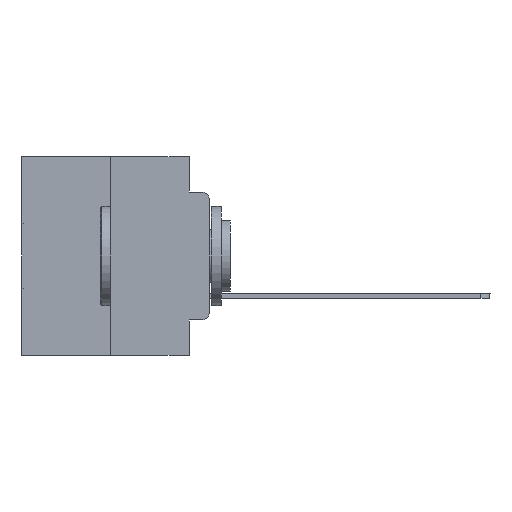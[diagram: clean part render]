
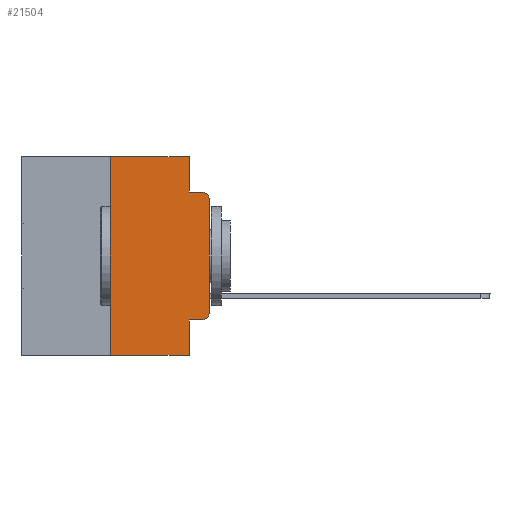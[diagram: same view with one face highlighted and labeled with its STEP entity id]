
A CAD part, left-side view. The second image highlights one B-rep face of the part: STEP entity #21504.
In plain terms, the highlighted planar face has unit normal (-1, 0, 0).
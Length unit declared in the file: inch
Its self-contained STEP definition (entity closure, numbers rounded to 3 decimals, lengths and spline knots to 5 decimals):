
#496 = VERTEX_POINT ( 'NONE', #14331 ) ;
#575 = EDGE_CURVE ( 'NONE', #27994, #496, #18154, .T. ) ;
#603 = ORIENTED_EDGE ( 'NONE', *, *, #17775, .T. ) ;
#1297 = CARTESIAN_POINT ( 'NONE',  ( 0., 0.473, 0. ) ) ;
#1309 = EDGE_CURVE ( 'NONE', #20811, #4275, #5692, .T. ) ;
#1399 = CARTESIAN_POINT ( 'NONE',  ( 0., 0.473, -0.5 ) ) ;
#2250 = EDGE_CURVE ( 'NONE', #29771, #3400, #20790, .T. ) ;
#2558 = CARTESIAN_POINT ( 'NONE',  ( 0., 0.02, -0.0885 ) ) ;
#2695 = VECTOR ( 'NONE', #11260, 39.37008 ) ;
#2806 = VECTOR ( 'NONE', #29273, 39.37008 ) ;
#2868 = ORIENTED_EDGE ( 'NONE', *, *, #575, .F. ) ;
#3094 = ORIENTED_EDGE ( 'NONE', *, *, #13580, .T. ) ;
#3380 = DIRECTION ( 'NONE',  ( 0., 0., -1. ) ) ;
#3400 = VERTEX_POINT ( 'NONE', #21935 ) ;
#3693 = DIRECTION ( 'NONE',  ( 0., -1., 0. ) ) ;
#4275 = VERTEX_POINT ( 'NONE', #17521 ) ;
#4934 = CARTESIAN_POINT ( 'NONE',  ( 0., 0.051, -0.0885 ) ) ;
#5692 = LINE ( 'NONE', #26639, #30234 ) ;
#5928 = DIRECTION ( 'NONE',  ( 0., 0., -1. ) ) ;
#6396 = VECTOR ( 'NONE', #3380, 39.37008 ) ;
#7435 = ORIENTED_EDGE ( 'NONE', *, *, #1309, .F. ) ;
#7499 = ORIENTED_EDGE ( 'NONE', *, *, #9379, .F. ) ;
#7923 = VERTEX_POINT ( 'NONE', #25984 ) ;
#8230 = CARTESIAN_POINT ( 'NONE',  ( 0., 0.051, 0. ) ) ;
#8682 = VERTEX_POINT ( 'NONE', #19244 ) ;
#9379 = EDGE_CURVE ( 'NONE', #8682, #20811, #21922, .T. ) ;
#9762 = ORIENTED_EDGE ( 'NONE', *, *, #10358, .F. ) ;
#10358 = EDGE_CURVE ( 'NONE', #18002, #27640, #24179, .T. ) ;
#10491 = LINE ( 'NONE', #1399, #2806 ) ;
#10536 = FACE_OUTER_BOUND ( 'NONE', #30091, .T. ) ;
#10923 = LINE ( 'NONE', #24789, #18863 ) ;
#11260 = DIRECTION ( 'NONE',  ( 0., 0., 1. ) ) ;
#11523 = ORIENTED_EDGE ( 'NONE', *, *, #27956, .F. ) ;
#13169 = CARTESIAN_POINT ( 'NONE',  ( 0., 0.051, -0.4115 ) ) ;
#13470 = DIRECTION ( 'NONE',  ( 0., 0., -1. ) ) ;
#13580 = EDGE_CURVE ( 'NONE', #27994, #7923, #10923, .T. ) ;
#14300 = VECTOR ( 'NONE', #17099, 39.37008 ) ;
#14331 = CARTESIAN_POINT ( 'NONE',  ( 0., 0.051, -0.5 ) ) ;
#14756 = AXIS2_PLACEMENT_3D ( 'NONE', #29560, #27397, #22765 ) ;
#15469 = LINE ( 'NONE', #8230, #17009 ) ;
#15713 = AXIS2_PLACEMENT_3D ( 'NONE', #1297, #24714, #24856 ) ;
#16041 = CARTESIAN_POINT ( 'NONE',  ( 0., 0., 0. ) ) ;
#17009 = VECTOR ( 'NONE', #13470, 39.37008 ) ;
#17099 = DIRECTION ( 'NONE',  ( 0., -1., 0. ) ) ;
#17191 = CIRCLE ( 'NONE', #19142, 0.02 ) ;
#17326 = DIRECTION ( 'NONE',  ( -1., 0., 0. ) ) ;
#17521 = CARTESIAN_POINT ( 'NONE',  ( 0., 0.051, 0. ) ) ;
#17775 = EDGE_CURVE ( 'NONE', #8682, #496, #10491, .T. ) ;
#18002 = VERTEX_POINT ( 'NONE', #26025 ) ;
#18154 = LINE ( 'NONE', #24467, #6396 ) ;
#18863 = VECTOR ( 'NONE', #3693, 39.37008 ) ;
#19142 = AXIS2_PLACEMENT_3D ( 'NONE', #22081, #17326, #5928 ) ;
#19244 = CARTESIAN_POINT ( 'NONE',  ( 0., 0.25, -0.5 ) ) ;
#19710 = DIRECTION ( 'NONE',  ( 0., -1., 0. ) ) ;
#20234 = PLANE ( 'NONE',  #15713 ) ;
#20790 = LINE ( 'NONE', #16041, #2695 ) ;
#20811 = VERTEX_POINT ( 'NONE', #27836 ) ;
#21425 = EDGE_CURVE ( 'NONE', #7923, #29771, #17191, .T. ) ;
#21504 = ADVANCED_FACE ( 'NONE', ( #10536 ), #20234, .F. ) ;
#21915 = EDGE_CURVE ( 'NONE', #3400, #27640, #29009, .T. ) ;
#21922 = LINE ( 'NONE', #22069, #29477 ) ;
#21935 = CARTESIAN_POINT ( 'NONE',  ( 0., 0., -0.1085 ) ) ;
#22069 = CARTESIAN_POINT ( 'NONE',  ( 0., 0.25, 0. ) ) ;
#22081 = CARTESIAN_POINT ( 'NONE',  ( 0., 0.02, -0.3915 ) ) ;
#22214 = DIRECTION ( 'NONE',  ( 0., 0., 1. ) ) ;
#22765 = DIRECTION ( 'NONE',  ( 0., 0., -1. ) ) ;
#23197 = ORIENTED_EDGE ( 'NONE', *, *, #21425, .T. ) ;
#24160 = CARTESIAN_POINT ( 'NONE',  ( 0., 0., -0.3915 ) ) ;
#24179 = LINE ( 'NONE', #4934, #14300 ) ;
#24467 = CARTESIAN_POINT ( 'NONE',  ( 0., 0.051, 0. ) ) ;
#24714 = DIRECTION ( 'NONE',  ( 1., 0., 0. ) ) ;
#24789 = CARTESIAN_POINT ( 'NONE',  ( 0., 0.051, -0.4115 ) ) ;
#24856 = DIRECTION ( 'NONE',  ( 0., 0., -1. ) ) ;
#25984 = CARTESIAN_POINT ( 'NONE',  ( 0., 0.02, -0.4115 ) ) ;
#26025 = CARTESIAN_POINT ( 'NONE',  ( 0., 0.051, -0.0885 ) ) ;
#26639 = CARTESIAN_POINT ( 'NONE',  ( 0., 0.473, 0. ) ) ;
#27397 = DIRECTION ( 'NONE',  ( -1., 0., 0. ) ) ;
#27640 = VERTEX_POINT ( 'NONE', #2558 ) ;
#27836 = CARTESIAN_POINT ( 'NONE',  ( 0., 0.25, 0. ) ) ;
#27956 = EDGE_CURVE ( 'NONE', #4275, #18002, #15469, .T. ) ;
#27994 = VERTEX_POINT ( 'NONE', #13169 ) ;
#29009 = CIRCLE ( 'NONE', #14756, 0.02 ) ;
#29273 = DIRECTION ( 'NONE',  ( 0., -1., 0. ) ) ;
#29302 = ORIENTED_EDGE ( 'NONE', *, *, #2250, .T. ) ;
#29345 = ORIENTED_EDGE ( 'NONE', *, *, #21915, .T. ) ;
#29477 = VECTOR ( 'NONE', #22214, 39.37008 ) ;
#29560 = CARTESIAN_POINT ( 'NONE',  ( 0., 0.02, -0.1085 ) ) ;
#29771 = VERTEX_POINT ( 'NONE', #24160 ) ;
#30091 = EDGE_LOOP ( 'NONE', ( #29302, #29345, #9762, #11523, #7435, #7499, #603, #2868, #3094, #23197 ) ) ;
#30234 = VECTOR ( 'NONE', #19710, 39.37008 ) ;
